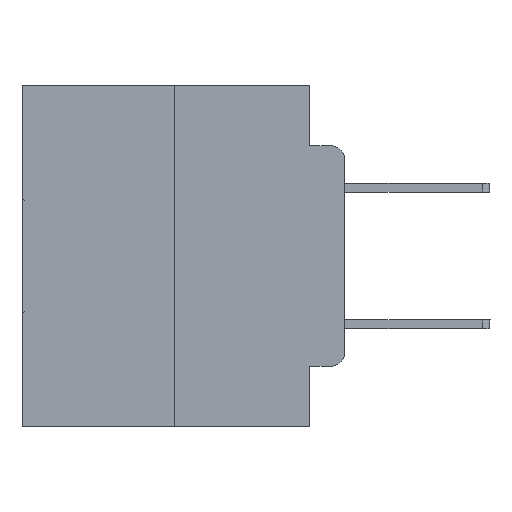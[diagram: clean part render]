
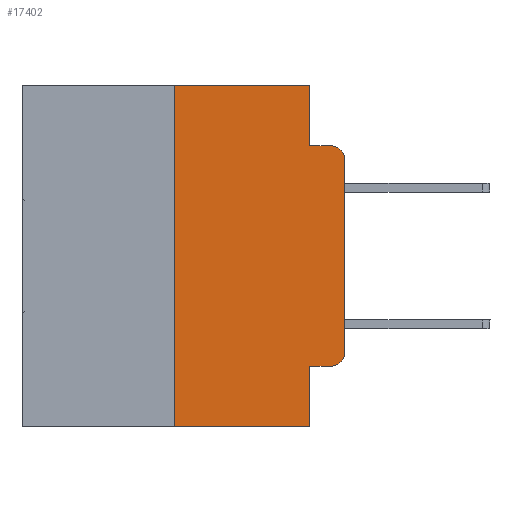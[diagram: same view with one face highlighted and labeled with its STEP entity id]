
A CAD part, left-side view. The second image highlights one B-rep face of the part: STEP entity #17402.
In plain terms, the highlighted planar face has unit normal (-1, 0, 0).
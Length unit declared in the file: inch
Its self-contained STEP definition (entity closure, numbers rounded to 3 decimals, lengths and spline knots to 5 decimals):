
#445 = EDGE_LOOP ( 'NONE', ( #4384, #29146, #11084, #10465, #6309, #28923, #8352, #14569, #29319, #7087 ) ) ;
#737 = LINE ( 'NONE', #7059, #22485 ) ;
#885 = PLANE ( 'NONE',  #4860 ) ;
#985 = DIRECTION ( 'NONE',  ( 1., 0., 0. ) ) ;
#1295 = CARTESIAN_POINT ( 'NONE',  ( 0., 0.051, -0.0885 ) ) ;
#2144 = AXIS2_PLACEMENT_3D ( 'NONE', #18719, #11027, #6118 ) ;
#2325 = LINE ( 'NONE', #25064, #6159 ) ;
#3170 = DIRECTION ( 'NONE',  ( 0., -1., 0. ) ) ;
#3343 = LINE ( 'NONE', #22825, #5655 ) ;
#3475 = VERTEX_POINT ( 'NONE', #29735 ) ;
#3751 = CARTESIAN_POINT ( 'NONE',  ( 0., 0.051, -0.4115 ) ) ;
#4384 = ORIENTED_EDGE ( 'NONE', *, *, #13419, .T. ) ;
#4662 = VERTEX_POINT ( 'NONE', #19372 ) ;
#4860 = AXIS2_PLACEMENT_3D ( 'NONE', #13113, #985, #5653 ) ;
#5264 = LINE ( 'NONE', #26546, #11737 ) ;
#5495 = EDGE_CURVE ( 'NONE', #16878, #7366, #3343, .T. ) ;
#5653 = DIRECTION ( 'NONE',  ( 0., 0., -1. ) ) ;
#5655 = VECTOR ( 'NONE', #29999, 39.37008 ) ;
#6118 = DIRECTION ( 'NONE',  ( 0., 0., -1. ) ) ;
#6159 = VECTOR ( 'NONE', #3170, 39.37008 ) ;
#6223 = DIRECTION ( 'NONE',  ( 0., 0., -1. ) ) ;
#6309 = ORIENTED_EDGE ( 'NONE', *, *, #31314, .F. ) ;
#7059 = CARTESIAN_POINT ( 'NONE',  ( 0., 0.473, -0.5 ) ) ;
#7087 = ORIENTED_EDGE ( 'NONE', *, *, #19854, .T. ) ;
#7366 = VERTEX_POINT ( 'NONE', #23123 ) ;
#7733 = VERTEX_POINT ( 'NONE', #10610 ) ;
#8113 = VERTEX_POINT ( 'NONE', #23928 ) ;
#8352 = ORIENTED_EDGE ( 'NONE', *, *, #28233, .T. ) ;
#8562 = VERTEX_POINT ( 'NONE', #25508 ) ;
#9878 = CARTESIAN_POINT ( 'NONE',  ( 0., 0.051, -0.0885 ) ) ;
#10149 = CIRCLE ( 'NONE', #2144, 0.02 ) ;
#10465 = ORIENTED_EDGE ( 'NONE', *, *, #24981, .F. ) ;
#10610 = CARTESIAN_POINT ( 'NONE',  ( 0., 0., -0.3915 ) ) ;
#11027 = DIRECTION ( 'NONE',  ( -1., 0., 0. ) ) ;
#11084 = ORIENTED_EDGE ( 'NONE', *, *, #21941, .F. ) ;
#11604 = VECTOR ( 'NONE', #23615, 39.37008 ) ;
#11709 = FACE_OUTER_BOUND ( 'NONE', #445, .T. ) ;
#11737 = VECTOR ( 'NONE', #16492, 39.37008 ) ;
#12504 = LINE ( 'NONE', #23096, #21670 ) ;
#12545 = VERTEX_POINT ( 'NONE', #28649 ) ;
#12556 = VERTEX_POINT ( 'NONE', #23723 ) ;
#13113 = CARTESIAN_POINT ( 'NONE',  ( 0., 0.473, 0. ) ) ;
#13133 = EDGE_CURVE ( 'NONE', #4662, #12545, #5264, .T. ) ;
#13419 = EDGE_CURVE ( 'NONE', #7733, #8113, #12504, .T. ) ;
#13579 = CARTESIAN_POINT ( 'NONE',  ( 0., 0.473, 0. ) ) ;
#14520 = DIRECTION ( 'NONE',  ( 0., 0., -1. ) ) ;
#14569 = ORIENTED_EDGE ( 'NONE', *, *, #5495, .F. ) ;
#16179 = AXIS2_PLACEMENT_3D ( 'NONE', #29176, #19370, #14520 ) ;
#16492 = DIRECTION ( 'NONE',  ( 0., 0., 1. ) ) ;
#16878 = VERTEX_POINT ( 'NONE', #3751 ) ;
#17402 = ADVANCED_FACE ( 'NONE', ( #11709 ), #885, .F. ) ;
#18430 = CIRCLE ( 'NONE', #16179, 0.02 ) ;
#18719 = CARTESIAN_POINT ( 'NONE',  ( 0., 0.02, -0.1085 ) ) ;
#19370 = DIRECTION ( 'NONE',  ( -1., 0., 0. ) ) ;
#19372 = CARTESIAN_POINT ( 'NONE',  ( 0., 0.25, -0.5 ) ) ;
#19854 = EDGE_CURVE ( 'NONE', #12556, #7733, #18430, .T. ) ;
#20260 = VECTOR ( 'NONE', #25841, 39.37008 ) ;
#20581 = EDGE_CURVE ( 'NONE', #16878, #12556, #2325, .T. ) ;
#21179 = LINE ( 'NONE', #26080, #28090 ) ;
#21670 = VECTOR ( 'NONE', #30354, 39.37008 ) ;
#21941 = EDGE_CURVE ( 'NONE', #22713, #8562, #28622, .T. ) ;
#22485 = VECTOR ( 'NONE', #28515, 39.37008 ) ;
#22713 = VERTEX_POINT ( 'NONE', #9878 ) ;
#22825 = CARTESIAN_POINT ( 'NONE',  ( 0., 0.051, 0. ) ) ;
#23096 = CARTESIAN_POINT ( 'NONE',  ( 0., 0., 0. ) ) ;
#23123 = CARTESIAN_POINT ( 'NONE',  ( 0., 0.051, -0.5 ) ) ;
#23615 = DIRECTION ( 'NONE',  ( 0., -1., 0. ) ) ;
#23723 = CARTESIAN_POINT ( 'NONE',  ( 0., 0.02, -0.4115 ) ) ;
#23928 = CARTESIAN_POINT ( 'NONE',  ( 0., 0., -0.1085 ) ) ;
#24923 = EDGE_CURVE ( 'NONE', #8113, #8562, #10149, .T. ) ;
#24981 = EDGE_CURVE ( 'NONE', #3475, #22713, #21179, .T. ) ;
#25064 = CARTESIAN_POINT ( 'NONE',  ( 0., 0.051, -0.4115 ) ) ;
#25508 = CARTESIAN_POINT ( 'NONE',  ( 0., 0.02, -0.0885 ) ) ;
#25841 = DIRECTION ( 'NONE',  ( 0., -1., 0. ) ) ;
#26080 = CARTESIAN_POINT ( 'NONE',  ( 0., 0.051, 0. ) ) ;
#26546 = CARTESIAN_POINT ( 'NONE',  ( 0., 0.25, 0. ) ) ;
#27678 = LINE ( 'NONE', #13579, #11604 ) ;
#28090 = VECTOR ( 'NONE', #6223, 39.37008 ) ;
#28233 = EDGE_CURVE ( 'NONE', #4662, #7366, #737, .T. ) ;
#28515 = DIRECTION ( 'NONE',  ( 0., -1., 0. ) ) ;
#28622 = LINE ( 'NONE', #1295, #20260 ) ;
#28649 = CARTESIAN_POINT ( 'NONE',  ( 0., 0.25, 0. ) ) ;
#28923 = ORIENTED_EDGE ( 'NONE', *, *, #13133, .F. ) ;
#29146 = ORIENTED_EDGE ( 'NONE', *, *, #24923, .T. ) ;
#29176 = CARTESIAN_POINT ( 'NONE',  ( 0., 0.02, -0.3915 ) ) ;
#29319 = ORIENTED_EDGE ( 'NONE', *, *, #20581, .T. ) ;
#29735 = CARTESIAN_POINT ( 'NONE',  ( 0., 0.051, 0. ) ) ;
#29999 = DIRECTION ( 'NONE',  ( 0., 0., -1. ) ) ;
#30354 = DIRECTION ( 'NONE',  ( 0., 0., 1. ) ) ;
#31314 = EDGE_CURVE ( 'NONE', #12545, #3475, #27678, .T. ) ;
